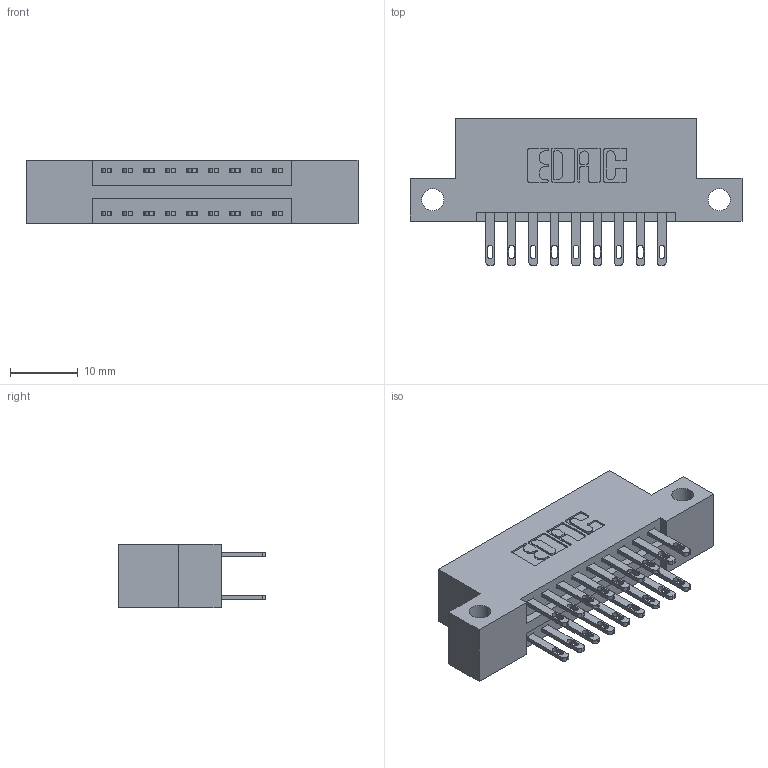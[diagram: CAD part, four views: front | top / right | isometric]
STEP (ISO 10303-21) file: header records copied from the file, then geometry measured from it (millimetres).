
FILE_DESCRIPTION (( 'STEP AP203' ), '1' );
FILE_NAME ('896-018-500-212.STEP', '2021-07-27T16:07:32', ( '' ), ( '' ), 'SwSTEP 2.0', 'SolidWorks 2020', '' );
FILE_SCHEMA (( 'CONFIG_CONTROL_DESIGN' ));
Length unit declared in the file: inch
Products named in the file (3): 345-292-001_345-293-100; 896-018-500-212; 846 Part_Flush Mounting Lugs - Side Mount
Assembly tree (19 placements, depth 2):
  896-018-500-212
    846 Part_Flush Mounting Lugs - Side Mount
    345-292-001_345-293-100  x18
Bounding box: 49.15 x 21.84 x 9.4 mm (x, y, z)
Volume: 4504 mm3; surface area: 5723.4 mm2
Topology: 19 solids, 19 shells, 986 faces, 2975 edges, 1982 vertices
Faces by surface type: plane 598, cylinder 388
Entity records: 10249 total; most frequent: CARTESIAN_POINT 1732, ORIENTED_EDGE 1666, DIRECTION 1581, EDGE_CURVE 833, LINE 661, VECTOR 661, VERTEX_POINT 554, AXIS2_PLACEMENT_3D 460
